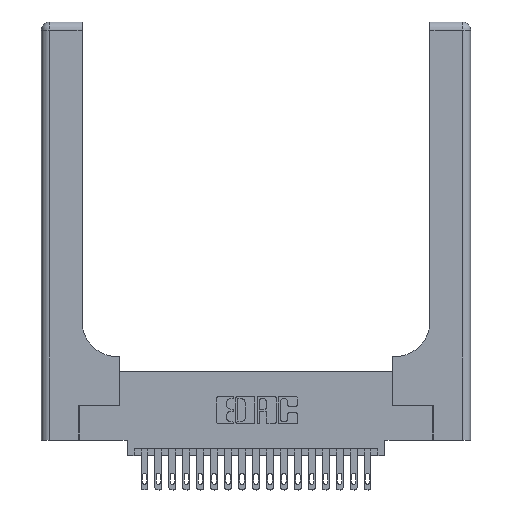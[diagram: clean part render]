
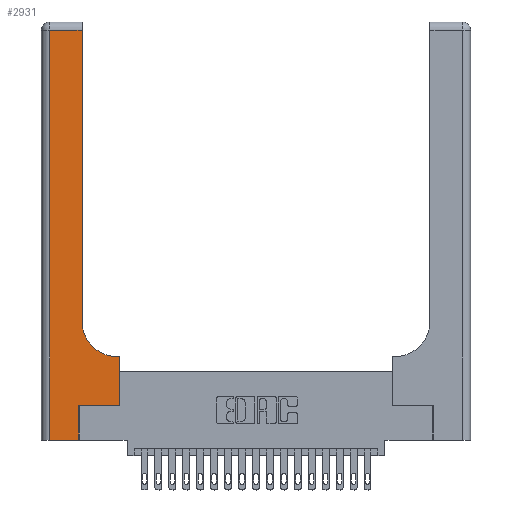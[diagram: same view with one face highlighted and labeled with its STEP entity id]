
A CAD part, top view. The second image highlights one B-rep face of the part: STEP entity #2931.
In plain terms, the highlighted planar face has unit normal (0, 0, 1).
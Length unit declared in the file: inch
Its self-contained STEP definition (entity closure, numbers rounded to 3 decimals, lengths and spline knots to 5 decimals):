
#26 = EDGE_CURVE ( 'NONE', #18087, #14771, #20524, .T. ) ;
#44 = ORIENTED_EDGE ( 'NONE', *, *, #10900, .T. ) ;
#89 = VERTEX_POINT ( 'NONE', #6381 ) ;
#269 = CARTESIAN_POINT ( 'NONE',  ( 0.2915, 2.94, 0.37 ) ) ;
#836 = VECTOR ( 'NONE', #9318, 39.37008 ) ;
#1395 = VERTEX_POINT ( 'NONE', #2811 ) ;
#1733 = VECTOR ( 'NONE', #16168, 39.37008 ) ;
#1832 = PLANE ( 'NONE',  #13702 ) ;
#1842 = CARTESIAN_POINT ( 'NONE',  ( 0., 0., 0.37 ) ) ;
#1897 = VERTEX_POINT ( 'NONE', #269 ) ;
#2154 = VECTOR ( 'NONE', #18955, 39.37008 ) ;
#2366 = EDGE_CURVE ( 'NONE', #6489, #18087, #6923, .T. ) ;
#2604 = EDGE_CURVE ( 'NONE', #89, #10898, #10134, .T. ) ;
#2633 = CARTESIAN_POINT ( 'NONE',  ( 0.06, 2.94, 0.37 ) ) ;
#2811 = CARTESIAN_POINT ( 'NONE',  ( 0.2915, 0.85, 0.37 ) ) ;
#2931 = ADVANCED_FACE ( 'NONE', ( #13586 ), #1832, .F. ) ;
#3023 = LINE ( 'NONE', #5854, #1733 ) ;
#3735 = ORIENTED_EDGE ( 'NONE', *, *, #16483, .T. ) ;
#3737 = DIRECTION ( 'NONE',  ( -1., 0., 0. ) ) ;
#4376 = CARTESIAN_POINT ( 'NONE',  ( 0.5415, 0.6, 0.37 ) ) ;
#5426 = LINE ( 'NONE', #5997, #21934 ) ;
#5448 = DIRECTION ( 'NONE',  ( 0., -1., 0. ) ) ;
#5769 = DIRECTION ( 'NONE',  ( 0., 0., -1. ) ) ;
#5849 = ORIENTED_EDGE ( 'NONE', *, *, #26, .T. ) ;
#5854 = CARTESIAN_POINT ( 'NONE',  ( 0., 2.94, 0.37 ) ) ;
#5997 = CARTESIAN_POINT ( 'NONE',  ( 0.5585, 0.25, 0.37 ) ) ;
#6360 = VECTOR ( 'NONE', #8598, 39.37008 ) ;
#6381 = CARTESIAN_POINT ( 'NONE',  ( 0.5585, 0.6, 0.37 ) ) ;
#6489 = VERTEX_POINT ( 'NONE', #17289 ) ;
#6545 = ORIENTED_EDGE ( 'NONE', *, *, #14384, .T. ) ;
#6923 = LINE ( 'NONE', #1842, #2154 ) ;
#7249 = EDGE_CURVE ( 'NONE', #1897, #12346, #3023, .T. ) ;
#7572 = LINE ( 'NONE', #17380, #16679 ) ;
#7611 = CARTESIAN_POINT ( 'NONE',  ( 0.269, 0., 0.37 ) ) ;
#8577 = CARTESIAN_POINT ( 'NONE',  ( 0.5585, 0.25, 0.37 ) ) ;
#8598 = DIRECTION ( 'NONE',  ( 0., 1., 0. ) ) ;
#8707 = CARTESIAN_POINT ( 'NONE',  ( 0.2915, 0.6, 0.37 ) ) ;
#9318 = DIRECTION ( 'NONE',  ( 0., 1., 0. ) ) ;
#9387 = DIRECTION ( 'NONE',  ( 1., 0., 0. ) ) ;
#10134 = LINE ( 'NONE', #8707, #18672 ) ;
#10880 = LINE ( 'NONE', #11111, #6360 ) ;
#10898 = VERTEX_POINT ( 'NONE', #4376 ) ;
#10900 = EDGE_CURVE ( 'NONE', #1395, #1897, #10880, .T. ) ;
#11111 = CARTESIAN_POINT ( 'NONE',  ( 0.2915, 3., 0.37 ) ) ;
#11764 = VECTOR ( 'NONE', #5448, 39.37008 ) ;
#12006 = LINE ( 'NONE', #17142, #11764 ) ;
#12280 = ORIENTED_EDGE ( 'NONE', *, *, #2604, .T. ) ;
#12346 = VERTEX_POINT ( 'NONE', #2633 ) ;
#13586 = FACE_OUTER_BOUND ( 'NONE', #14632, .T. ) ;
#13702 = AXIS2_PLACEMENT_3D ( 'NONE', #19098, #19399, #21306 ) ;
#13946 = ORIENTED_EDGE ( 'NONE', *, *, #14203, .T. ) ;
#14203 = EDGE_CURVE ( 'NONE', #10898, #1395, #18265, .T. ) ;
#14384 = EDGE_CURVE ( 'NONE', #14771, #17836, #7572, .T. ) ;
#14480 = CARTESIAN_POINT ( 'NONE',  ( 0.269, 0., 0.37 ) ) ;
#14632 = EDGE_LOOP ( 'NONE', ( #44, #19087, #15173, #20143, #5849, #6545, #3735, #12280, #13946 ) ) ;
#14771 = VERTEX_POINT ( 'NONE', #20025 ) ;
#15173 = ORIENTED_EDGE ( 'NONE', *, *, #17587, .T. ) ;
#16168 = DIRECTION ( 'NONE',  ( -1., 0., 0. ) ) ;
#16290 = DIRECTION ( 'NONE',  ( 1., 0., 0. ) ) ;
#16483 = EDGE_CURVE ( 'NONE', #17836, #89, #5426, .T. ) ;
#16679 = VECTOR ( 'NONE', #9387, 39.37008 ) ;
#17142 = CARTESIAN_POINT ( 'NONE',  ( 0.06, 3., 0.37 ) ) ;
#17289 = CARTESIAN_POINT ( 'NONE',  ( 0.06, 0., 0.37 ) ) ;
#17380 = CARTESIAN_POINT ( 'NONE',  ( 0.269, 0.25, 0.37 ) ) ;
#17587 = EDGE_CURVE ( 'NONE', #12346, #6489, #12006, .T. ) ;
#17836 = VERTEX_POINT ( 'NONE', #8577 ) ;
#17938 = DIRECTION ( 'NONE',  ( 0., 1., 0. ) ) ;
#18087 = VERTEX_POINT ( 'NONE', #14480 ) ;
#18265 = CIRCLE ( 'NONE', #21822, 0.25 ) ;
#18672 = VECTOR ( 'NONE', #3737, 39.37008 ) ;
#18955 = DIRECTION ( 'NONE',  ( 1., 0., 0. ) ) ;
#19087 = ORIENTED_EDGE ( 'NONE', *, *, #7249, .T. ) ;
#19098 = CARTESIAN_POINT ( 'NONE',  ( 0., 3., 0.37 ) ) ;
#19399 = DIRECTION ( 'NONE',  ( 0., 0., -1. ) ) ;
#20025 = CARTESIAN_POINT ( 'NONE',  ( 0.269, 0.25, 0.37 ) ) ;
#20143 = ORIENTED_EDGE ( 'NONE', *, *, #2366, .T. ) ;
#20524 = LINE ( 'NONE', #7611, #836 ) ;
#21306 = DIRECTION ( 'NONE',  ( -1., 0., 0. ) ) ;
#21337 = CARTESIAN_POINT ( 'NONE',  ( 0.5415, 0.85, 0.37 ) ) ;
#21822 = AXIS2_PLACEMENT_3D ( 'NONE', #21337, #5769, #16290 ) ;
#21934 = VECTOR ( 'NONE', #17938, 39.37008 ) ;
